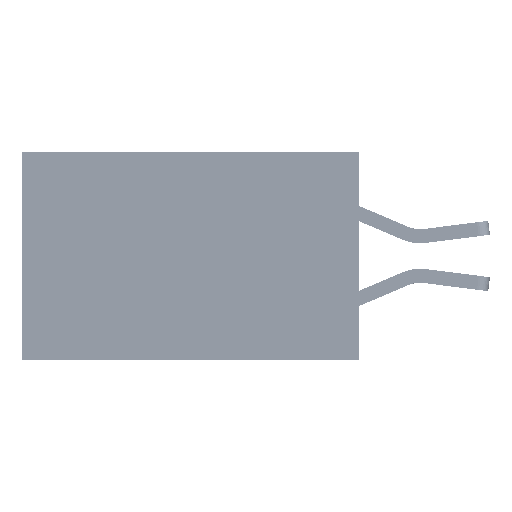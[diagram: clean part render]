
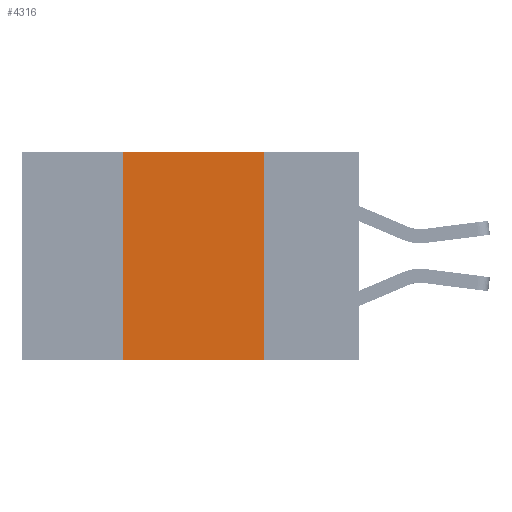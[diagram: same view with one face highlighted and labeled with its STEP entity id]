
A CAD part, left-side view. The second image highlights one B-rep face of the part: STEP entity #4316.
In plain terms, the highlighted planar face has unit normal (-1, 0, 0).
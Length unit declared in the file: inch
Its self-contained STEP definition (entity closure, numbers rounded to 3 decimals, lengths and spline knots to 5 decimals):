
#2284 = FACE_OUTER_BOUND ( 'NONE', #41719, .T. ) ;
#4316 = ADVANCED_FACE ( 'NONE', ( #2284 ), #32520, .F. ) ;
#4743 = LINE ( 'NONE', #8353, #39583 ) ;
#5862 = EDGE_CURVE ( 'NONE', #8661, #30969, #30287, .T. ) ;
#6667 = DIRECTION ( 'NONE',  ( 0., -1., 0. ) ) ;
#8353 = CARTESIAN_POINT ( 'NONE',  ( 0., 0.42, 0. ) ) ;
#8661 = VERTEX_POINT ( 'NONE', #31462 ) ;
#9586 = VECTOR ( 'NONE', #34650, 39.37008 ) ;
#10811 = CARTESIAN_POINT ( 'NONE',  ( 0., 0.6, -0.37 ) ) ;
#14315 = EDGE_CURVE ( 'NONE', #29679, #30969, #22744, .T. ) ;
#16694 = CARTESIAN_POINT ( 'NONE',  ( 0., 0.17, 0. ) ) ;
#18076 = ORIENTED_EDGE ( 'NONE', *, *, #14315, .F. ) ;
#18730 = ORIENTED_EDGE ( 'NONE', *, *, #34410, .F. ) ;
#20373 = ORIENTED_EDGE ( 'NONE', *, *, #5862, .T. ) ;
#21863 = DIRECTION ( 'NONE',  ( 0., 0., -1. ) ) ;
#22744 = LINE ( 'NONE', #16694, #43802 ) ;
#24994 = CARTESIAN_POINT ( 'NONE',  ( 0., 0.42, 0. ) ) ;
#25073 = DIRECTION ( 'NONE',  ( 1., 0., 0. ) ) ;
#27464 = CARTESIAN_POINT ( 'NONE',  ( 0., 0.17, 0. ) ) ;
#28491 = CARTESIAN_POINT ( 'NONE',  ( 0., 0.6, 0. ) ) ;
#29679 = VERTEX_POINT ( 'NONE', #27464 ) ;
#30287 = LINE ( 'NONE', #10811, #36367 ) ;
#30969 = VERTEX_POINT ( 'NONE', #43316 ) ;
#31108 = CARTESIAN_POINT ( 'NONE',  ( 0., 0.6, 0. ) ) ;
#31462 = CARTESIAN_POINT ( 'NONE',  ( 0., 0.42, -0.37 ) ) ;
#32520 = PLANE ( 'NONE',  #36641 ) ;
#33122 = DIRECTION ( 'NONE',  ( 0., 0., 1. ) ) ;
#34410 = EDGE_CURVE ( 'NONE', #35172, #29679, #35057, .T. ) ;
#34650 = DIRECTION ( 'NONE',  ( 0., -1., 0. ) ) ;
#35057 = LINE ( 'NONE', #31108, #9586 ) ;
#35172 = VERTEX_POINT ( 'NONE', #24994 ) ;
#36367 = VECTOR ( 'NONE', #6667, 39.37008 ) ;
#36641 = AXIS2_PLACEMENT_3D ( 'NONE', #28491, #25073, #21863 ) ;
#38020 = DIRECTION ( 'NONE',  ( 0., 0., -1. ) ) ;
#39251 = EDGE_CURVE ( 'NONE', #8661, #35172, #4743, .T. ) ;
#39583 = VECTOR ( 'NONE', #33122, 39.37008 ) ;
#41719 = EDGE_LOOP ( 'NONE', ( #18076, #18730, #42631, #20373 ) ) ;
#42631 = ORIENTED_EDGE ( 'NONE', *, *, #39251, .F. ) ;
#43316 = CARTESIAN_POINT ( 'NONE',  ( 0., 0.17, -0.37 ) ) ;
#43802 = VECTOR ( 'NONE', #38020, 39.37008 ) ;
